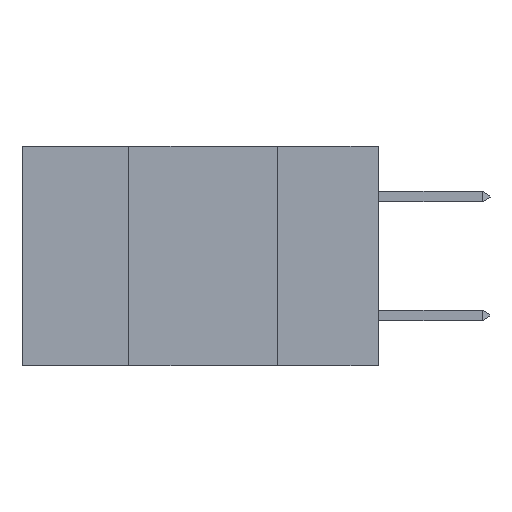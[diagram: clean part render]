
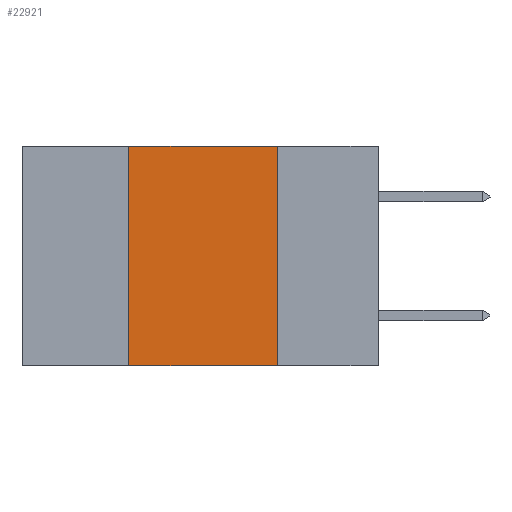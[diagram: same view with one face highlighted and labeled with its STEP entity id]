
A CAD part, left-side view. The second image highlights one B-rep face of the part: STEP entity #22921.
In plain terms, the highlighted planar face has unit normal (-1, 0, 0).
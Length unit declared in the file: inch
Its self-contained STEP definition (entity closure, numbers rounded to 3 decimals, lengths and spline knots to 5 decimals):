
#113 = VERTEX_POINT ( 'NONE', #6768 ) ;
#230 = EDGE_CURVE ( 'NONE', #20828, #13148, #20528, .T. ) ;
#273 = ORIENTED_EDGE ( 'NONE', *, *, #230, .F. ) ;
#737 = DIRECTION ( 'NONE',  ( 0., -1., 0. ) ) ;
#2170 = VECTOR ( 'NONE', #2639, 39.37008 ) ;
#2639 = DIRECTION ( 'NONE',  ( 0., 0., 1. ) ) ;
#3996 = FACE_OUTER_BOUND ( 'NONE', #18623, .T. ) ;
#4055 = CARTESIAN_POINT ( 'NONE',  ( 0., 0.42, -0.37 ) ) ;
#4872 = AXIS2_PLACEMENT_3D ( 'NONE', #26396, #12856, #28654 ) ;
#6263 = DIRECTION ( 'NONE',  ( 0., 0., -1. ) ) ;
#6768 = CARTESIAN_POINT ( 'NONE',  ( 0., 0.17, 0. ) ) ;
#8034 = EDGE_CURVE ( 'NONE', #20828, #9548, #8926, .T. ) ;
#8926 = LINE ( 'NONE', #28126, #25647 ) ;
#9548 = VERTEX_POINT ( 'NONE', #24787 ) ;
#10514 = PLANE ( 'NONE',  #4872 ) ;
#11836 = VECTOR ( 'NONE', #24531, 39.37008 ) ;
#12856 = DIRECTION ( 'NONE',  ( 1., 0., 0. ) ) ;
#13148 = VERTEX_POINT ( 'NONE', #25288 ) ;
#14816 = EDGE_CURVE ( 'NONE', #113, #9548, #17254, .T. ) ;
#16530 = VECTOR ( 'NONE', #6263, 39.37008 ) ;
#17254 = LINE ( 'NONE', #29017, #16530 ) ;
#17326 = CARTESIAN_POINT ( 'NONE',  ( 0., 0.42, 0. ) ) ;
#18623 = EDGE_LOOP ( 'NONE', ( #25715, #23289, #273, #26085 ) ) ;
#19416 = EDGE_CURVE ( 'NONE', #13148, #113, #23917, .T. ) ;
#20528 = LINE ( 'NONE', #17326, #2170 ) ;
#20828 = VERTEX_POINT ( 'NONE', #4055 ) ;
#22281 = CARTESIAN_POINT ( 'NONE',  ( 0., 0.6, 0. ) ) ;
#22921 = ADVANCED_FACE ( 'NONE', ( #3996 ), #10514, .F. ) ;
#23289 = ORIENTED_EDGE ( 'NONE', *, *, #19416, .F. ) ;
#23917 = LINE ( 'NONE', #22281, #11836 ) ;
#24531 = DIRECTION ( 'NONE',  ( 0., -1., 0. ) ) ;
#24787 = CARTESIAN_POINT ( 'NONE',  ( 0., 0.17, -0.37 ) ) ;
#25288 = CARTESIAN_POINT ( 'NONE',  ( 0., 0.42, 0. ) ) ;
#25647 = VECTOR ( 'NONE', #737, 39.37008 ) ;
#25715 = ORIENTED_EDGE ( 'NONE', *, *, #14816, .F. ) ;
#26085 = ORIENTED_EDGE ( 'NONE', *, *, #8034, .T. ) ;
#26396 = CARTESIAN_POINT ( 'NONE',  ( 0., 0.6, 0. ) ) ;
#28126 = CARTESIAN_POINT ( 'NONE',  ( 0., 0.6, -0.37 ) ) ;
#28654 = DIRECTION ( 'NONE',  ( 0., 0., -1. ) ) ;
#29017 = CARTESIAN_POINT ( 'NONE',  ( 0., 0.17, 0. ) ) ;
